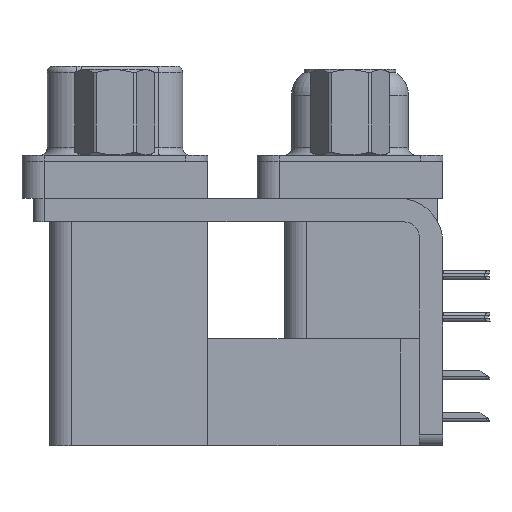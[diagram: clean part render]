
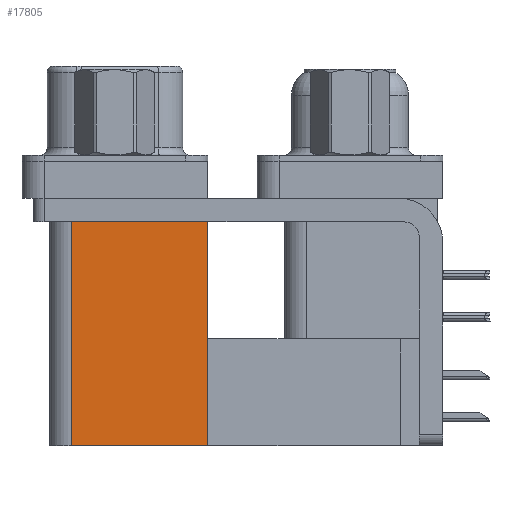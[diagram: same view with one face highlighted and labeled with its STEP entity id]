
A CAD part, left-side view. The second image highlights one B-rep face of the part: STEP entity #17805.
In plain terms, the highlighted planar face has unit normal (-1, 0, 0).
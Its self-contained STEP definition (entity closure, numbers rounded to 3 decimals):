
#2416 = ORIENTED_EDGE ( 'NONE', *, *, #21977, .T. ) ;
#4078 = LINE ( 'NONE', #42338, #38627 ) ;
#7333 = CARTESIAN_POINT ( 'NONE',  ( 3.765, 9.6, -2.5 ) ) ;
#7879 = ORIENTED_EDGE ( 'NONE', *, *, #25224, .T. ) ;
#7928 = AXIS2_PLACEMENT_3D ( 'NONE', #33137, #48195, #25951 ) ;
#8496 = DIRECTION ( 'NONE',  ( 0., 0., 1. ) ) ;
#10759 = LINE ( 'NONE', #14691, #26837 ) ;
#12936 = VERTEX_POINT ( 'NONE', #44169 ) ;
#14388 = CARTESIAN_POINT ( 'NONE',  ( 3.765, 9.6, -2.5 ) ) ;
#14691 = CARTESIAN_POINT ( 'NONE',  ( 3.765, 9.6, -19.2 ) ) ;
#17028 = ORIENTED_EDGE ( 'NONE', *, *, #46984, .F. ) ;
#17805 = ADVANCED_FACE ( 'NONE', ( #22744 ), #29637, .F. ) ;
#19523 = LINE ( 'NONE', #42519, #35780 ) ;
#21566 = LINE ( 'NONE', #14388, #28096 ) ;
#21977 = EDGE_CURVE ( 'NONE', #44567, #29612, #21566, .T. ) ;
#22744 = FACE_OUTER_BOUND ( 'NONE', #26557, .T. ) ;
#25224 = EDGE_CURVE ( 'NONE', #12936, #44567, #10759, .T. ) ;
#25951 = DIRECTION ( 'NONE',  ( 0., 0., -1. ) ) ;
#26557 = EDGE_LOOP ( 'NONE', ( #2416, #17028, #27555, #7879 ) ) ;
#26837 = VECTOR ( 'NONE', #37953, 1000. ) ;
#27555 = ORIENTED_EDGE ( 'NONE', *, *, #42542, .F. ) ;
#28096 = VECTOR ( 'NONE', #29218, 1000. ) ;
#28289 = VERTEX_POINT ( 'NONE', #37321 ) ;
#29218 = DIRECTION ( 'NONE',  ( 0., 1., 0. ) ) ;
#29612 = VERTEX_POINT ( 'NONE', #43051 ) ;
#29637 = PLANE ( 'NONE',  #7928 ) ;
#33137 = CARTESIAN_POINT ( 'NONE',  ( 3.765, 9.6, -19.2 ) ) ;
#35780 = VECTOR ( 'NONE', #45989, 1000. ) ;
#37321 = CARTESIAN_POINT ( 'NONE',  ( 3.765, 18.8, -19.2 ) ) ;
#37953 = DIRECTION ( 'NONE',  ( 0., 0., 1. ) ) ;
#38627 = VECTOR ( 'NONE', #8496, 1000. ) ;
#42338 = CARTESIAN_POINT ( 'NONE',  ( 3.765, 18.8, -19.2 ) ) ;
#42519 = CARTESIAN_POINT ( 'NONE',  ( 3.765, 9.6, -19.2 ) ) ;
#42542 = EDGE_CURVE ( 'NONE', #12936, #28289, #19523, .T. ) ;
#43051 = CARTESIAN_POINT ( 'NONE',  ( 3.765, 18.8, -2.5 ) ) ;
#44169 = CARTESIAN_POINT ( 'NONE',  ( 3.765, 9.6, -19.2 ) ) ;
#44567 = VERTEX_POINT ( 'NONE', #7333 ) ;
#45989 = DIRECTION ( 'NONE',  ( 0., 1., 0. ) ) ;
#46984 = EDGE_CURVE ( 'NONE', #28289, #29612, #4078, .T. ) ;
#48195 = DIRECTION ( 'NONE',  ( 1., 0., 0. ) ) ;
